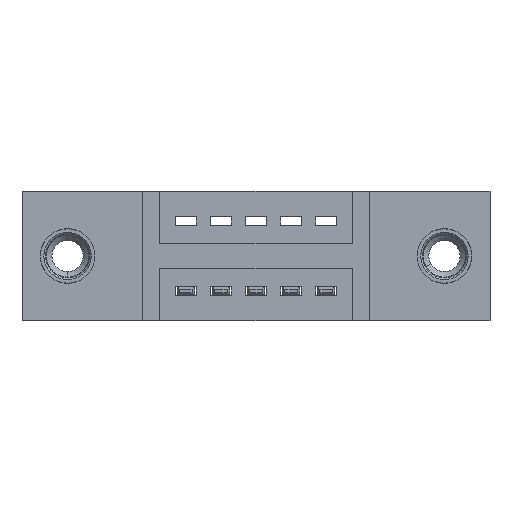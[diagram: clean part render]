
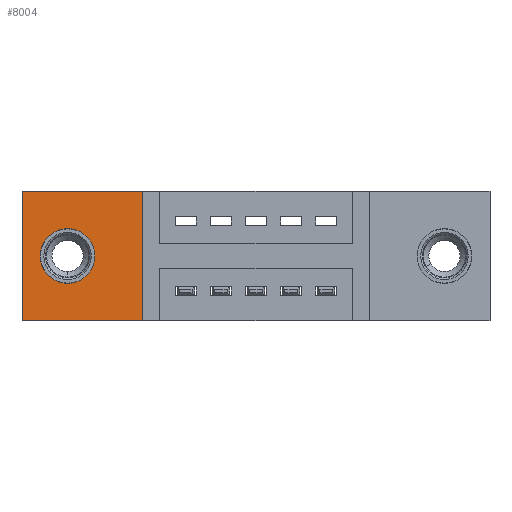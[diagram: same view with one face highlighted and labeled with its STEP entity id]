
A CAD part, front view. The second image highlights one B-rep face of the part: STEP entity #8004.
In plain terms, the highlighted planar face has unit normal (0, -1, 0).
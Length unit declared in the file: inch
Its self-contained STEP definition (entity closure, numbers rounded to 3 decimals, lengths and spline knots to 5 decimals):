
#130 = ORIENTED_EDGE ( 'NONE', *, *, #6149, .F. ) ;
#304 = EDGE_LOOP ( 'NONE', ( #5878, #130 ) ) ;
#351 = VECTOR ( 'NONE', #7715, 39.37008 ) ;
#496 = CARTESIAN_POINT ( 'NONE',  ( 0., 0.17, -0.37 ) ) ;
#806 = VECTOR ( 'NONE', #7491, 39.37008 ) ;
#842 = CARTESIAN_POINT ( 'NONE',  ( 0., 0.17, 0. ) ) ;
#898 = EDGE_CURVE ( 'NONE', #7643, #5919, #3477, .T. ) ;
#1388 = AXIS2_PLACEMENT_3D ( 'NONE', #6301, #3265, #4103 ) ;
#1523 = EDGE_CURVE ( 'NONE', #8647, #7643, #5954, .T. ) ;
#1601 = ORIENTED_EDGE ( 'NONE', *, *, #898, .T. ) ;
#1730 = CARTESIAN_POINT ( 'NONE',  ( 0., 0.17, 0. ) ) ;
#1797 = CIRCLE ( 'NONE', #1388, 0.078 ) ;
#2063 = VERTEX_POINT ( 'NONE', #8530 ) ;
#2094 = ORIENTED_EDGE ( 'NONE', *, *, #1523, .T. ) ;
#2337 = AXIS2_PLACEMENT_3D ( 'NONE', #8876, #7249, #3447 ) ;
#2365 = LINE ( 'NONE', #6949, #351 ) ;
#2646 = AXIS2_PLACEMENT_3D ( 'NONE', #8474, #5372, #9316 ) ;
#2715 = PLANE ( 'NONE',  #2337 ) ;
#2718 = CARTESIAN_POINT ( 'NONE',  ( 0.13, 0.17, -0.107 ) ) ;
#2768 = VERTEX_POINT ( 'NONE', #496 ) ;
#2964 = CARTESIAN_POINT ( 'NONE',  ( 0.3425, 0.17, -0.37 ) ) ;
#3077 = CIRCLE ( 'NONE', #2646, 0.078 ) ;
#3265 = DIRECTION ( 'NONE',  ( 0., -1., 0. ) ) ;
#3381 = DIRECTION ( 'NONE',  ( 0., 0., 1. ) ) ;
#3447 = DIRECTION ( 'NONE',  ( 0., 0., -1. ) ) ;
#3477 = LINE ( 'NONE', #1730, #9359 ) ;
#4103 = DIRECTION ( 'NONE',  ( 0., 0., -1. ) ) ;
#4158 = VECTOR ( 'NONE', #3381, 39.37008 ) ;
#4346 = FACE_BOUND ( 'NONE', #304, .T. ) ;
#5372 = DIRECTION ( 'NONE',  ( 0., -1., 0. ) ) ;
#5532 = DIRECTION ( 'NONE',  ( -1., 0., 0. ) ) ;
#5878 = ORIENTED_EDGE ( 'NONE', *, *, #5935, .F. ) ;
#5898 = FACE_OUTER_BOUND ( 'NONE', #7335, .T. ) ;
#5919 = VERTEX_POINT ( 'NONE', #842 ) ;
#5935 = EDGE_CURVE ( 'NONE', #9236, #2063, #1797, .T. ) ;
#5954 = LINE ( 'NONE', #8782, #4158 ) ;
#6149 = EDGE_CURVE ( 'NONE', #2063, #9236, #3077, .T. ) ;
#6301 = CARTESIAN_POINT ( 'NONE',  ( 0.13, 0.17, -0.185 ) ) ;
#6602 = EDGE_CURVE ( 'NONE', #2768, #8647, #2365, .T. ) ;
#6691 = CARTESIAN_POINT ( 'NONE',  ( 0., 0.17, 0. ) ) ;
#6949 = CARTESIAN_POINT ( 'NONE',  ( 0., 0.17, -0.37 ) ) ;
#7249 = DIRECTION ( 'NONE',  ( 0., -1., 0. ) ) ;
#7335 = EDGE_LOOP ( 'NONE', ( #8098, #9334, #2094, #1601 ) ) ;
#7491 = DIRECTION ( 'NONE',  ( 0., 0., -1. ) ) ;
#7581 = EDGE_CURVE ( 'NONE', #5919, #2768, #9533, .T. ) ;
#7643 = VERTEX_POINT ( 'NONE', #7911 ) ;
#7715 = DIRECTION ( 'NONE',  ( 1., 0., 0. ) ) ;
#7911 = CARTESIAN_POINT ( 'NONE',  ( 0.3425, 0.17, 0. ) ) ;
#8004 = ADVANCED_FACE ( 'NONE', ( #4346, #5898 ), #2715, .T. ) ;
#8098 = ORIENTED_EDGE ( 'NONE', *, *, #7581, .T. ) ;
#8474 = CARTESIAN_POINT ( 'NONE',  ( 0.13, 0.17, -0.185 ) ) ;
#8530 = CARTESIAN_POINT ( 'NONE',  ( 0.13, 0.17, -0.263 ) ) ;
#8647 = VERTEX_POINT ( 'NONE', #2964 ) ;
#8782 = CARTESIAN_POINT ( 'NONE',  ( 0.3425, 0.17, 0. ) ) ;
#8876 = CARTESIAN_POINT ( 'NONE',  ( 0., 0.17, -0.37 ) ) ;
#9236 = VERTEX_POINT ( 'NONE', #2718 ) ;
#9316 = DIRECTION ( 'NONE',  ( 0., 0., -1. ) ) ;
#9334 = ORIENTED_EDGE ( 'NONE', *, *, #6602, .T. ) ;
#9359 = VECTOR ( 'NONE', #5532, 39.37008 ) ;
#9533 = LINE ( 'NONE', #6691, #806 ) ;
